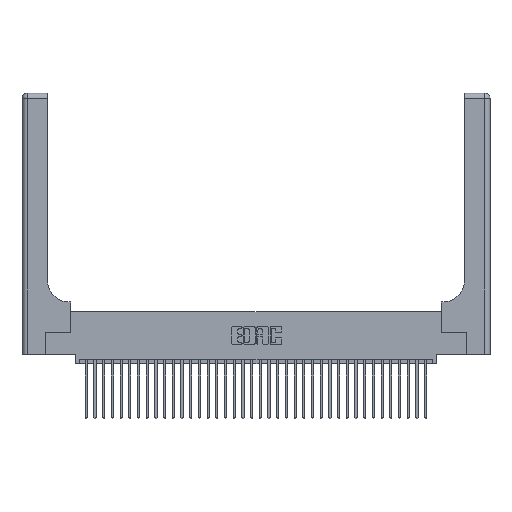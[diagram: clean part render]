
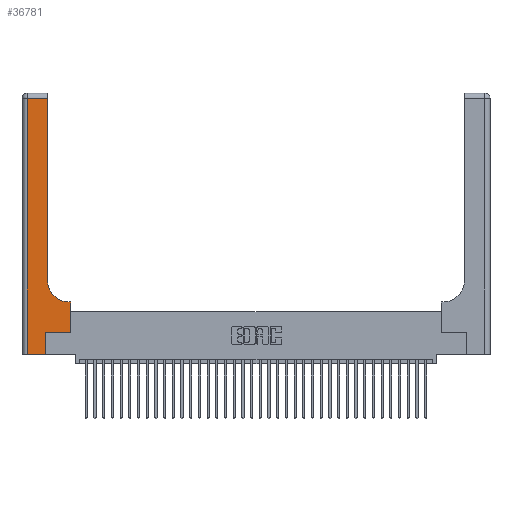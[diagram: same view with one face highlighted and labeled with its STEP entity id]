
A CAD part, top view. The second image highlights one B-rep face of the part: STEP entity #36781.
In plain terms, the highlighted planar face has unit normal (0, 0, 1).
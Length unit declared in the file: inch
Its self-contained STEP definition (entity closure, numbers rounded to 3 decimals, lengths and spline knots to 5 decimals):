
#680 = VECTOR ( 'NONE', #36115, 39.37008 ) ;
#707 = EDGE_CURVE ( 'NONE', #10672, #32502, #27699, .T. ) ;
#1558 = LINE ( 'NONE', #1990, #28045 ) ;
#1658 = CARTESIAN_POINT ( 'NONE',  ( 0.2915, 2.94, 0.37 ) ) ;
#1913 = CARTESIAN_POINT ( 'NONE',  ( 0.5415, 0.85, 0.37 ) ) ;
#1990 = CARTESIAN_POINT ( 'NONE',  ( 0.06, 3., 0.37 ) ) ;
#2273 = DIRECTION ( 'NONE',  ( 0., 1., 0. ) ) ;
#2294 = VECTOR ( 'NONE', #26106, 39.37008 ) ;
#3233 = ORIENTED_EDGE ( 'NONE', *, *, #25037, .T. ) ;
#3381 = ORIENTED_EDGE ( 'NONE', *, *, #7084, .T. ) ;
#3764 = CARTESIAN_POINT ( 'NONE',  ( 0., 0., 0.37 ) ) ;
#4568 = LINE ( 'NONE', #3764, #34101 ) ;
#4576 = DIRECTION ( 'NONE',  ( -1., 0., 0. ) ) ;
#4935 = CARTESIAN_POINT ( 'NONE',  ( 0.5415, 0.6, 0.37 ) ) ;
#6122 = ORIENTED_EDGE ( 'NONE', *, *, #18838, .T. ) ;
#7031 = VECTOR ( 'NONE', #26343, 39.37008 ) ;
#7084 = EDGE_CURVE ( 'NONE', #14318, #7526, #1558, .T. ) ;
#7307 = DIRECTION ( 'NONE',  ( 1., 0., 0. ) ) ;
#7526 = VERTEX_POINT ( 'NONE', #8199 ) ;
#7544 = ORIENTED_EDGE ( 'NONE', *, *, #29132, .T. ) ;
#8199 = CARTESIAN_POINT ( 'NONE',  ( 0.06, 0., 0.37 ) ) ;
#9303 = LINE ( 'NONE', #10149, #680 ) ;
#9401 = ORIENTED_EDGE ( 'NONE', *, *, #22575, .T. ) ;
#9975 = DIRECTION ( 'NONE',  ( -1., 0., 0. ) ) ;
#10033 = CARTESIAN_POINT ( 'NONE',  ( 0.2915, 3., 0.37 ) ) ;
#10149 = CARTESIAN_POINT ( 'NONE',  ( 0.5585, 0.25, 0.37 ) ) ;
#10672 = VERTEX_POINT ( 'NONE', #33243 ) ;
#10981 = VECTOR ( 'NONE', #9975, 39.37008 ) ;
#11359 = AXIS2_PLACEMENT_3D ( 'NONE', #13485, #30561, #33447 ) ;
#11551 = ORIENTED_EDGE ( 'NONE', *, *, #707, .T. ) ;
#11619 = EDGE_CURVE ( 'NONE', #26428, #17529, #15112, .T. ) ;
#12544 = VECTOR ( 'NONE', #2273, 39.37008 ) ;
#13485 = CARTESIAN_POINT ( 'NONE',  ( 0., 3., 0.37 ) ) ;
#13742 = PLANE ( 'NONE',  #11359 ) ;
#14144 = FACE_OUTER_BOUND ( 'NONE', #32049, .T. ) ;
#14318 = VERTEX_POINT ( 'NONE', #27943 ) ;
#15112 = LINE ( 'NONE', #26074, #7031 ) ;
#15225 = LINE ( 'NONE', #21064, #2294 ) ;
#16536 = ORIENTED_EDGE ( 'NONE', *, *, #21925, .T. ) ;
#17335 = ORIENTED_EDGE ( 'NONE', *, *, #11619, .T. ) ;
#17369 = CIRCLE ( 'NONE', #20136, 0.25 ) ;
#17529 = VERTEX_POINT ( 'NONE', #18321 ) ;
#17599 = LINE ( 'NONE', #29899, #10981 ) ;
#18321 = CARTESIAN_POINT ( 'NONE',  ( 0.5585, 0.25, 0.37 ) ) ;
#18838 = EDGE_CURVE ( 'NONE', #28524, #24881, #32203, .T. ) ;
#20136 = AXIS2_PLACEMENT_3D ( 'NONE', #1913, #30290, #7307 ) ;
#21064 = CARTESIAN_POINT ( 'NONE',  ( 0.269, 0., 0.37 ) ) ;
#21925 = EDGE_CURVE ( 'NONE', #7526, #25812, #4568, .T. ) ;
#22426 = CARTESIAN_POINT ( 'NONE',  ( 0.269, 0., 0.37 ) ) ;
#22575 = EDGE_CURVE ( 'NONE', #25812, #26428, #15225, .T. ) ;
#24452 = CARTESIAN_POINT ( 'NONE',  ( 0.2915, 0.6, 0.37 ) ) ;
#24881 = VERTEX_POINT ( 'NONE', #1658 ) ;
#25037 = EDGE_CURVE ( 'NONE', #17529, #10672, #9303, .T. ) ;
#25812 = VERTEX_POINT ( 'NONE', #22426 ) ;
#26074 = CARTESIAN_POINT ( 'NONE',  ( 0.269, 0.25, 0.37 ) ) ;
#26106 = DIRECTION ( 'NONE',  ( 0., 1., 0. ) ) ;
#26343 = DIRECTION ( 'NONE',  ( 1., 0., 0. ) ) ;
#26428 = VERTEX_POINT ( 'NONE', #27220 ) ;
#26753 = DIRECTION ( 'NONE',  ( 1., 0., 0. ) ) ;
#27220 = CARTESIAN_POINT ( 'NONE',  ( 0.269, 0.25, 0.37 ) ) ;
#27699 = LINE ( 'NONE', #24452, #30365 ) ;
#27943 = CARTESIAN_POINT ( 'NONE',  ( 0.06, 2.94, 0.37 ) ) ;
#28045 = VECTOR ( 'NONE', #30890, 39.37008 ) ;
#28524 = VERTEX_POINT ( 'NONE', #31288 ) ;
#29132 = EDGE_CURVE ( 'NONE', #24881, #14318, #17599, .T. ) ;
#29899 = CARTESIAN_POINT ( 'NONE',  ( 0., 2.94, 0.37 ) ) ;
#30290 = DIRECTION ( 'NONE',  ( 0., 0., -1. ) ) ;
#30365 = VECTOR ( 'NONE', #4576, 39.37008 ) ;
#30561 = DIRECTION ( 'NONE',  ( 0., 0., -1. ) ) ;
#30890 = DIRECTION ( 'NONE',  ( 0., -1., 0. ) ) ;
#31288 = CARTESIAN_POINT ( 'NONE',  ( 0.2915, 0.85, 0.37 ) ) ;
#32049 = EDGE_LOOP ( 'NONE', ( #6122, #7544, #3381, #16536, #9401, #17335, #3233, #11551, #36975 ) ) ;
#32203 = LINE ( 'NONE', #10033, #12544 ) ;
#32502 = VERTEX_POINT ( 'NONE', #4935 ) ;
#33243 = CARTESIAN_POINT ( 'NONE',  ( 0.5585, 0.6, 0.37 ) ) ;
#33447 = DIRECTION ( 'NONE',  ( -1., 0., 0. ) ) ;
#34101 = VECTOR ( 'NONE', #26753, 39.37008 ) ;
#34786 = EDGE_CURVE ( 'NONE', #32502, #28524, #17369, .T. ) ;
#36115 = DIRECTION ( 'NONE',  ( 0., 1., 0. ) ) ;
#36781 = ADVANCED_FACE ( 'NONE', ( #14144 ), #13742, .F. ) ;
#36975 = ORIENTED_EDGE ( 'NONE', *, *, #34786, .T. ) ;
